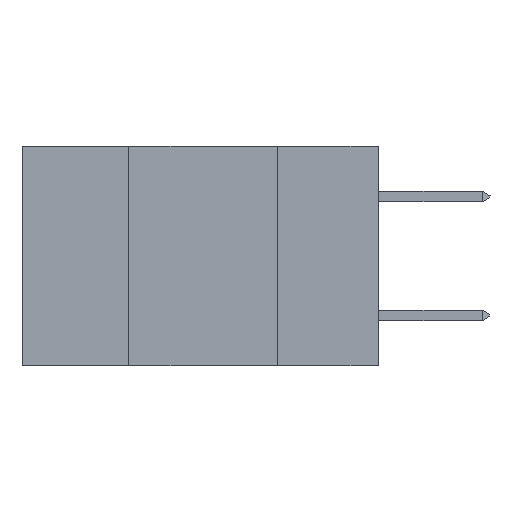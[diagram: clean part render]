
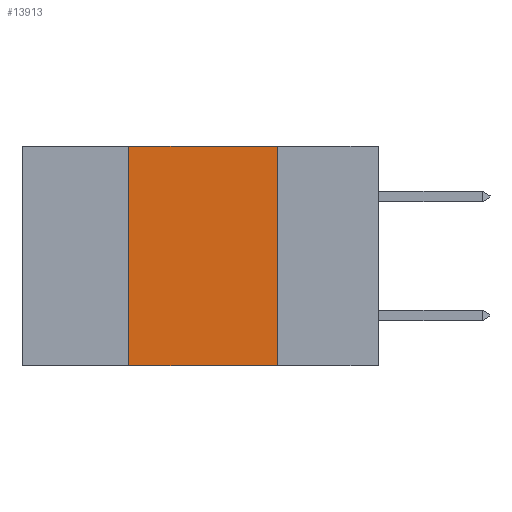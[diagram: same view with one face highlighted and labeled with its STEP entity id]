
A CAD part, left-side view. The second image highlights one B-rep face of the part: STEP entity #13913.
In plain terms, the highlighted planar face has unit normal (-1, 0, 0).
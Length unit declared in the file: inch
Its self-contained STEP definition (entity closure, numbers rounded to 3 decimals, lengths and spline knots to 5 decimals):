
#338 = CARTESIAN_POINT ( 'NONE',  ( 0., 0.17, -0.37 ) ) ;
#848 = CARTESIAN_POINT ( 'NONE',  ( 0., 0.6, 0. ) ) ;
#1235 = CARTESIAN_POINT ( 'NONE',  ( 0., 0.17, -0.37 ) ) ;
#1840 = CARTESIAN_POINT ( 'NONE',  ( 0., 0.42, 0. ) ) ;
#1848 = DIRECTION ( 'NONE',  ( 0., -1., 0. ) ) ;
#3145 = CARTESIAN_POINT ( 'NONE',  ( 0., 0.6, 0. ) ) ;
#3506 = ORIENTED_EDGE ( 'NONE', *, *, #16569, .F. ) ;
#3563 = EDGE_LOOP ( 'NONE', ( #5259, #3506, #7833, #13154 ) ) ;
#5251 = VECTOR ( 'NONE', #6460, 39.37008 ) ;
#5259 = ORIENTED_EDGE ( 'NONE', *, *, #14341, .F. ) ;
#5831 = VECTOR ( 'NONE', #7354, 39.37008 ) ;
#6156 = VERTEX_POINT ( 'NONE', #1840 ) ;
#6423 = LINE ( 'NONE', #15449, #12746 ) ;
#6460 = DIRECTION ( 'NONE',  ( 0., 0., -1. ) ) ;
#7232 = LINE ( 'NONE', #8420, #16260 ) ;
#7354 = DIRECTION ( 'NONE',  ( 0., -1., 0. ) ) ;
#7829 = PLANE ( 'NONE',  #9802 ) ;
#7833 = ORIENTED_EDGE ( 'NONE', *, *, #12715, .F. ) ;
#7855 = CARTESIAN_POINT ( 'NONE',  ( 0., 0.42, -0.37 ) ) ;
#8420 = CARTESIAN_POINT ( 'NONE',  ( 0., 0.6, -0.37 ) ) ;
#9802 = AXIS2_PLACEMENT_3D ( 'NONE', #848, #16602, #13675 ) ;
#10198 = VERTEX_POINT ( 'NONE', #338 ) ;
#11248 = CARTESIAN_POINT ( 'NONE',  ( 0., 0.17, 0. ) ) ;
#11405 = DIRECTION ( 'NONE',  ( 0., 0., 1. ) ) ;
#11507 = VERTEX_POINT ( 'NONE', #7855 ) ;
#12715 = EDGE_CURVE ( 'NONE', #11507, #6156, #6423, .T. ) ;
#12746 = VECTOR ( 'NONE', #11405, 39.37008 ) ;
#13154 = ORIENTED_EDGE ( 'NONE', *, *, #13394, .T. ) ;
#13394 = EDGE_CURVE ( 'NONE', #11507, #10198, #7232, .T. ) ;
#13675 = DIRECTION ( 'NONE',  ( 0., 0., -1. ) ) ;
#13913 = ADVANCED_FACE ( 'NONE', ( #15335 ), #7829, .F. ) ;
#14341 = EDGE_CURVE ( 'NONE', #14856, #10198, #15394, .T. ) ;
#14704 = LINE ( 'NONE', #3145, #5831 ) ;
#14856 = VERTEX_POINT ( 'NONE', #11248 ) ;
#15335 = FACE_OUTER_BOUND ( 'NONE', #3563, .T. ) ;
#15394 = LINE ( 'NONE', #1235, #5251 ) ;
#15449 = CARTESIAN_POINT ( 'NONE',  ( 0., 0.42, -0.37 ) ) ;
#16260 = VECTOR ( 'NONE', #1848, 39.37008 ) ;
#16569 = EDGE_CURVE ( 'NONE', #6156, #14856, #14704, .T. ) ;
#16602 = DIRECTION ( 'NONE',  ( 1., 0., 0. ) ) ;
